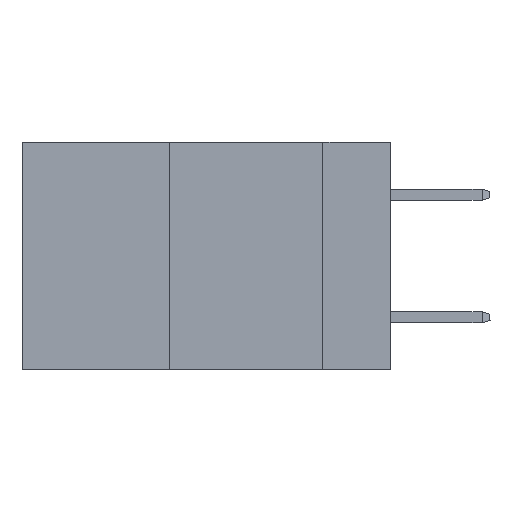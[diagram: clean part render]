
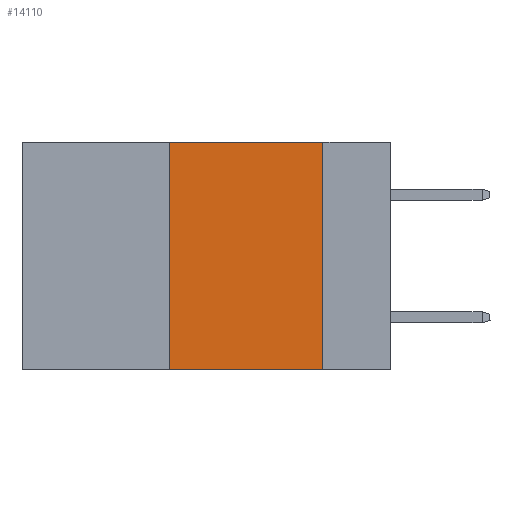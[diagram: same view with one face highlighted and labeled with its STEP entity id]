
A CAD part, left-side view. The second image highlights one B-rep face of the part: STEP entity #14110.
In plain terms, the highlighted planar face has unit normal (-1, 0, 0).
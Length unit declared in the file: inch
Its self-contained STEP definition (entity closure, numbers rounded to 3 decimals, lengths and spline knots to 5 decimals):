
#614 = CARTESIAN_POINT ( 'NONE',  ( 0., 0.11, -0.37 ) ) ;
#726 = CARTESIAN_POINT ( 'NONE',  ( 0., 0.11, 0. ) ) ;
#1443 = LINE ( 'NONE', #2982, #5118 ) ;
#1609 = CARTESIAN_POINT ( 'NONE',  ( 0., 0.6, 0. ) ) ;
#1712 = VECTOR ( 'NONE', #14450, 39.37008 ) ;
#1735 = LINE ( 'NONE', #15927, #1712 ) ;
#2409 = ORIENTED_EDGE ( 'NONE', *, *, #10650, .F. ) ;
#2938 = VECTOR ( 'NONE', #14819, 39.37008 ) ;
#2982 = CARTESIAN_POINT ( 'NONE',  ( 0., 0.11, 0. ) ) ;
#3215 = LINE ( 'NONE', #15601, #16116 ) ;
#4041 = EDGE_LOOP ( 'NONE', ( #2409, #5340, #15438, #12204 ) ) ;
#4869 = CARTESIAN_POINT ( 'NONE',  ( 0., 0.36, -0.37 ) ) ;
#5118 = VECTOR ( 'NONE', #16869, 39.37008 ) ;
#5340 = ORIENTED_EDGE ( 'NONE', *, *, #8946, .F. ) ;
#5532 = CARTESIAN_POINT ( 'NONE',  ( 0., 0.36, 0. ) ) ;
#7967 = CARTESIAN_POINT ( 'NONE',  ( 0., 0.6, -0.37 ) ) ;
#8946 = EDGE_CURVE ( 'NONE', #16967, #14126, #3215, .T. ) ;
#9439 = LINE ( 'NONE', #7967, #2938 ) ;
#9544 = FACE_OUTER_BOUND ( 'NONE', #4041, .T. ) ;
#10085 = PLANE ( 'NONE',  #10841 ) ;
#10650 = EDGE_CURVE ( 'NONE', #14126, #12517, #1443, .T. ) ;
#10841 = AXIS2_PLACEMENT_3D ( 'NONE', #1609, #11347, #12841 ) ;
#11347 = DIRECTION ( 'NONE',  ( 1., 0., 0. ) ) ;
#12204 = ORIENTED_EDGE ( 'NONE', *, *, #17648, .T. ) ;
#12517 = VERTEX_POINT ( 'NONE', #614 ) ;
#12841 = DIRECTION ( 'NONE',  ( 0., 0., -1. ) ) ;
#14110 = ADVANCED_FACE ( 'NONE', ( #9544 ), #10085, .F. ) ;
#14126 = VERTEX_POINT ( 'NONE', #726 ) ;
#14450 = DIRECTION ( 'NONE',  ( 0., 0., 1. ) ) ;
#14738 = EDGE_CURVE ( 'NONE', #17810, #16967, #1735, .T. ) ;
#14819 = DIRECTION ( 'NONE',  ( 0., -1., 0. ) ) ;
#15438 = ORIENTED_EDGE ( 'NONE', *, *, #14738, .F. ) ;
#15601 = CARTESIAN_POINT ( 'NONE',  ( 0., 0.6, 0. ) ) ;
#15927 = CARTESIAN_POINT ( 'NONE',  ( 0., 0.36, 0. ) ) ;
#16116 = VECTOR ( 'NONE', #17132, 39.37008 ) ;
#16869 = DIRECTION ( 'NONE',  ( 0., 0., -1. ) ) ;
#16967 = VERTEX_POINT ( 'NONE', #5532 ) ;
#17132 = DIRECTION ( 'NONE',  ( 0., -1., 0. ) ) ;
#17648 = EDGE_CURVE ( 'NONE', #17810, #12517, #9439, .T. ) ;
#17810 = VERTEX_POINT ( 'NONE', #4869 ) ;
